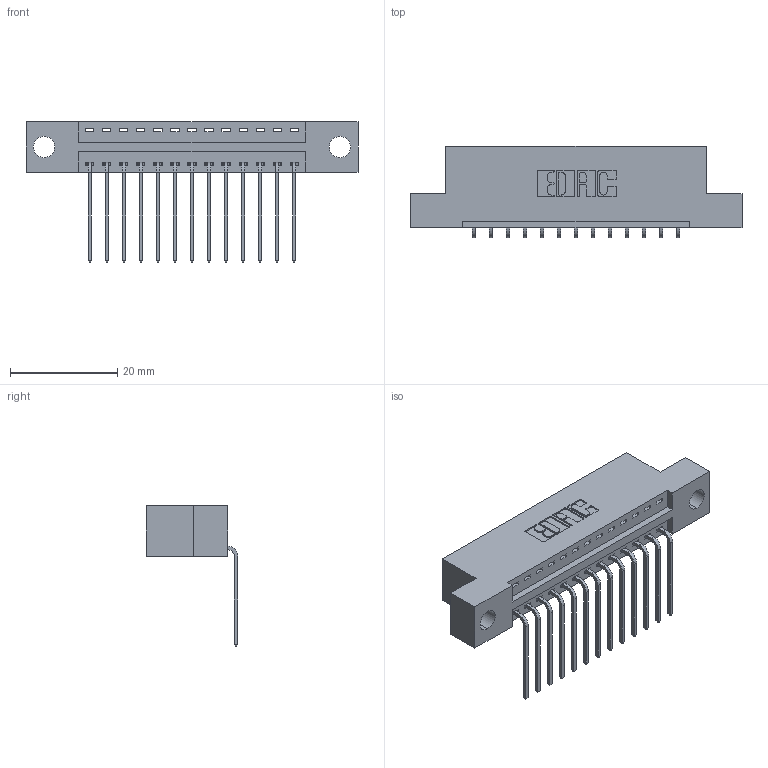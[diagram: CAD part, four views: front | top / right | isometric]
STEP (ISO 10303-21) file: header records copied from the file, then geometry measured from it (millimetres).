
FILE_DESCRIPTION (( 'STEP AP203' ), '1' );
FILE_NAME ('346-013-559-104.STEP', '2022-05-05T05:16:26', ( '' ), ( '' ), 'SwSTEP 2.0', 'SolidWorks 2020', '' );
FILE_SCHEMA (( 'CONFIG_CONTROL_DESIGN' ));
Length unit declared in the file: inch
Products named in the file (3): 346 Part_Flush Mounting Lugs - 0.156 Dia-TH; 345-292-001_558 559 Tail - 1; 346-013-559-104
Assembly tree (14 placements, depth 2):
  346-013-559-104
    346 Part_Flush Mounting Lugs - 0.156 Dia-TH
    345-292-001_558 559 Tail - 1  x13
Bounding box: 61.85 x 17.08 x 26.16 mm (x, y, z)
Volume: 5657.9 mm3; surface area: 6854.3 mm2
Topology: 14 solids, 14 shells, 916 faces, 2731 edges, 1802 vertices
Faces by surface type: plane 636, cylinder 280
Entity records: 12475 total; most frequent: CARTESIAN_POINT 2157, ORIENTED_EDGE 2102, DIRECTION 1937, EDGE_CURVE 1051, VECTOR 867, LINE 867, VERTEX_POINT 698, AXIS2_PLACEMENT_3D 535
